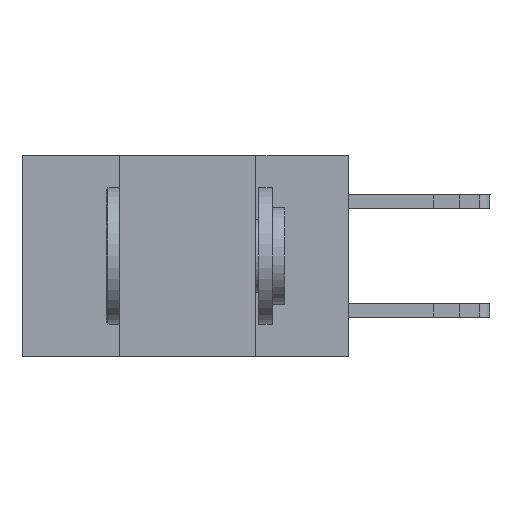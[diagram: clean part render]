
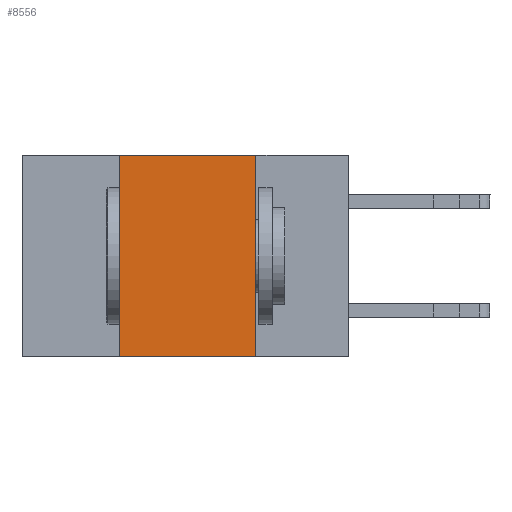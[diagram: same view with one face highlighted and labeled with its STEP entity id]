
A CAD part, left-side view. The second image highlights one B-rep face of the part: STEP entity #8556.
In plain terms, the highlighted planar face has unit normal (-1, 0, 0).
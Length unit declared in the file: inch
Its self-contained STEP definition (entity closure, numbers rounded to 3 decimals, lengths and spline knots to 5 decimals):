
#2044 = ORIENTED_EDGE ( 'NONE', *, *, #11225, .F. ) ;
#3552 = CARTESIAN_POINT ( 'NONE',  ( 0., 0.42, -0.37 ) ) ;
#3643 = CARTESIAN_POINT ( 'NONE',  ( 0., 0.6, 0. ) ) ;
#3844 = LINE ( 'NONE', #20291, #6263 ) ;
#3969 = CARTESIAN_POINT ( 'NONE',  ( 0., 0.42, 0. ) ) ;
#6064 = VERTEX_POINT ( 'NONE', #7519 ) ;
#6263 = VECTOR ( 'NONE', #20504, 39.37008 ) ;
#6278 = VERTEX_POINT ( 'NONE', #3552 ) ;
#6938 = DIRECTION ( 'NONE',  ( 0., -1., 0. ) ) ;
#7519 = CARTESIAN_POINT ( 'NONE',  ( 0., 0.17, -0.37 ) ) ;
#7917 = EDGE_CURVE ( 'NONE', #9380, #20392, #8801, .T. ) ;
#8550 = CARTESIAN_POINT ( 'NONE',  ( 0., 0.6, 0. ) ) ;
#8556 = ADVANCED_FACE ( 'NONE', ( #11973 ), #10204, .F. ) ;
#8801 = LINE ( 'NONE', #3643, #12455 ) ;
#9026 = LINE ( 'NONE', #3969, #21619 ) ;
#9380 = VERTEX_POINT ( 'NONE', #20653 ) ;
#9994 = LINE ( 'NONE', #11429, #20438 ) ;
#10055 = AXIS2_PLACEMENT_3D ( 'NONE', #8550, #12829, #15709 ) ;
#10204 = PLANE ( 'NONE',  #10055 ) ;
#10342 = EDGE_CURVE ( 'NONE', #20392, #6064, #3844, .T. ) ;
#10711 = ORIENTED_EDGE ( 'NONE', *, *, #7917, .F. ) ;
#11225 = EDGE_CURVE ( 'NONE', #6278, #9380, #9026, .T. ) ;
#11429 = CARTESIAN_POINT ( 'NONE',  ( 0., 0.6, -0.37 ) ) ;
#11461 = EDGE_CURVE ( 'NONE', #6278, #6064, #9994, .T. ) ;
#11921 = DIRECTION ( 'NONE',  ( 0., 0., 1. ) ) ;
#11973 = FACE_OUTER_BOUND ( 'NONE', #14024, .T. ) ;
#12455 = VECTOR ( 'NONE', #6938, 39.37008 ) ;
#12829 = DIRECTION ( 'NONE',  ( 1., 0., 0. ) ) ;
#14024 = EDGE_LOOP ( 'NONE', ( #18850, #10711, #2044, #15008 ) ) ;
#15008 = ORIENTED_EDGE ( 'NONE', *, *, #11461, .T. ) ;
#15053 = DIRECTION ( 'NONE',  ( 0., -1., 0. ) ) ;
#15709 = DIRECTION ( 'NONE',  ( 0., 0., -1. ) ) ;
#18850 = ORIENTED_EDGE ( 'NONE', *, *, #10342, .F. ) ;
#20291 = CARTESIAN_POINT ( 'NONE',  ( 0., 0.17, 0. ) ) ;
#20392 = VERTEX_POINT ( 'NONE', #21244 ) ;
#20438 = VECTOR ( 'NONE', #15053, 39.37008 ) ;
#20504 = DIRECTION ( 'NONE',  ( 0., 0., -1. ) ) ;
#20653 = CARTESIAN_POINT ( 'NONE',  ( 0., 0.42, 0. ) ) ;
#21244 = CARTESIAN_POINT ( 'NONE',  ( 0., 0.17, 0. ) ) ;
#21619 = VECTOR ( 'NONE', #11921, 39.37008 ) ;
